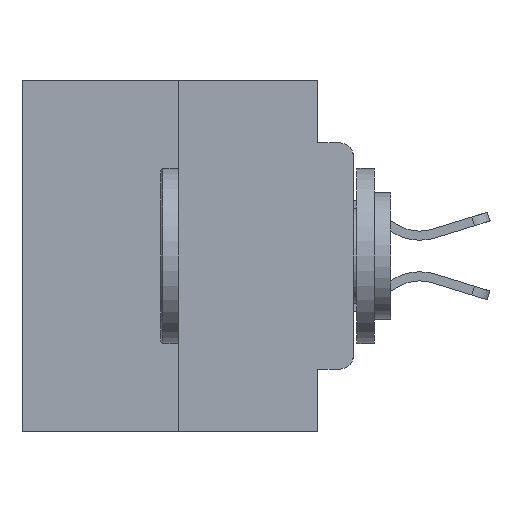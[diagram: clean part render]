
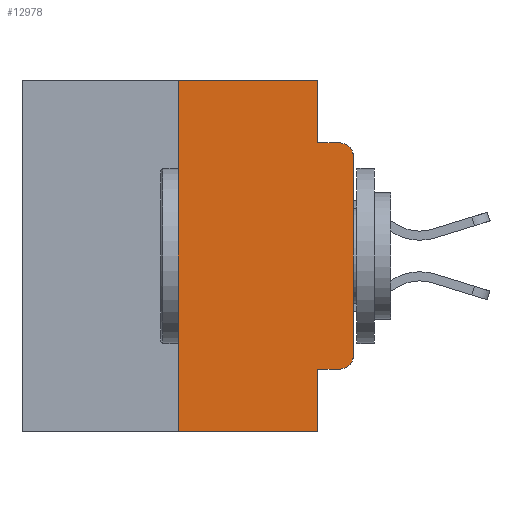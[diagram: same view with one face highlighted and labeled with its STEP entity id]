
A CAD part, left-side view. The second image highlights one B-rep face of the part: STEP entity #12978.
In plain terms, the highlighted planar face has unit normal (-1, 0, 0).
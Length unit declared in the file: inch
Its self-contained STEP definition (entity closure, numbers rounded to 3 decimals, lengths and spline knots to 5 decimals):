
#45 = ORIENTED_EDGE ( 'NONE', *, *, #5260, .T. ) ;
#410 = EDGE_CURVE ( 'NONE', #4877, #18952, #23578, .T. ) ;
#663 = VERTEX_POINT ( 'NONE', #10787 ) ;
#1080 = CARTESIAN_POINT ( 'NONE',  ( 0., 0.02, -0.4115 ) ) ;
#1214 = CIRCLE ( 'NONE', #4079, 0.02 ) ;
#1266 = DIRECTION ( 'NONE',  ( 0., 0., -1. ) ) ;
#1281 = CARTESIAN_POINT ( 'NONE',  ( 0., 0.25, 0. ) ) ;
#1569 = ORIENTED_EDGE ( 'NONE', *, *, #19447, .F. ) ;
#2007 = ORIENTED_EDGE ( 'NONE', *, *, #410, .T. ) ;
#2140 = VERTEX_POINT ( 'NONE', #1281 ) ;
#2347 = VECTOR ( 'NONE', #6789, 39.37008 ) ;
#2609 = ORIENTED_EDGE ( 'NONE', *, *, #10534, .F. ) ;
#2623 = VECTOR ( 'NONE', #26717, 39.37008 ) ;
#2697 = DIRECTION ( 'NONE',  ( 0., -1., 0. ) ) ;
#2991 = CARTESIAN_POINT ( 'NONE',  ( 0., 0.02, -0.1085 ) ) ;
#3119 = ORIENTED_EDGE ( 'NONE', *, *, #18502, .F. ) ;
#3158 = LINE ( 'NONE', #25580, #23714 ) ;
#3335 = CARTESIAN_POINT ( 'NONE',  ( 0., 0.02, -0.0885 ) ) ;
#3342 = VERTEX_POINT ( 'NONE', #7476 ) ;
#3512 = EDGE_LOOP ( 'NONE', ( #21358, #22064, #22658, #17281, #3119, #2609, #2007, #1569, #45, #16520 ) ) ;
#3519 = DIRECTION ( 'NONE',  ( 1., 0., 0. ) ) ;
#3778 = EDGE_CURVE ( 'NONE', #18759, #14320, #3158, .T. ) ;
#4079 = AXIS2_PLACEMENT_3D ( 'NONE', #2991, #17925, #5199 ) ;
#4141 = EDGE_CURVE ( 'NONE', #25461, #663, #26878, .T. ) ;
#4877 = VERTEX_POINT ( 'NONE', #12364 ) ;
#5199 = DIRECTION ( 'NONE',  ( 0., 0., -1. ) ) ;
#5260 = EDGE_CURVE ( 'NONE', #12381, #22173, #23355, .T. ) ;
#5715 = CARTESIAN_POINT ( 'NONE',  ( 0., 0.25, 0. ) ) ;
#5802 = CARTESIAN_POINT ( 'NONE',  ( 0., 0.473, -0.5 ) ) ;
#5827 = CARTESIAN_POINT ( 'NONE',  ( 0., 0.051, 0. ) ) ;
#5860 = CARTESIAN_POINT ( 'NONE',  ( 0., 0.051, -0.0885 ) ) ;
#6789 = DIRECTION ( 'NONE',  ( 0., -1., 0. ) ) ;
#7265 = VECTOR ( 'NONE', #7481, 39.37008 ) ;
#7355 = VECTOR ( 'NONE', #18394, 39.37008 ) ;
#7476 = CARTESIAN_POINT ( 'NONE',  ( 0., 0.051, 0. ) ) ;
#7481 = DIRECTION ( 'NONE',  ( 0., -1., 0. ) ) ;
#8270 = EDGE_CURVE ( 'NONE', #22173, #25461, #11747, .T. ) ;
#8455 = LINE ( 'NONE', #5827, #2623 ) ;
#8773 = CARTESIAN_POINT ( 'NONE',  ( 0., 0.02, -0.3915 ) ) ;
#9856 = VECTOR ( 'NONE', #2697, 39.37008 ) ;
#10022 = CARTESIAN_POINT ( 'NONE',  ( 0., 0.473, 0. ) ) ;
#10534 = EDGE_CURVE ( 'NONE', #4877, #2140, #18562, .T. ) ;
#10787 = CARTESIAN_POINT ( 'NONE',  ( 0., 0., -0.1085 ) ) ;
#10939 = DIRECTION ( 'NONE',  ( 0., 0., -1. ) ) ;
#11041 = EDGE_CURVE ( 'NONE', #663, #14320, #1214, .T. ) ;
#11046 = DIRECTION ( 'NONE',  ( 0., -1., 0. ) ) ;
#11747 = CIRCLE ( 'NONE', #19338, 0.02 ) ;
#12364 = CARTESIAN_POINT ( 'NONE',  ( 0., 0.25, -0.5 ) ) ;
#12381 = VERTEX_POINT ( 'NONE', #14376 ) ;
#12978 = ADVANCED_FACE ( 'NONE', ( #24630 ), #16344, .F. ) ;
#13913 = CARTESIAN_POINT ( 'NONE',  ( 0., 0.051, -0.4115 ) ) ;
#14320 = VERTEX_POINT ( 'NONE', #3335 ) ;
#14376 = CARTESIAN_POINT ( 'NONE',  ( 0., 0.051, -0.4115 ) ) ;
#14987 = CARTESIAN_POINT ( 'NONE',  ( 0., 0.051, -0.5 ) ) ;
#15224 = VECTOR ( 'NONE', #16331, 39.37008 ) ;
#16158 = EDGE_CURVE ( 'NONE', #3342, #18759, #24354, .T. ) ;
#16269 = CARTESIAN_POINT ( 'NONE',  ( 0., 0.051, 0. ) ) ;
#16331 = DIRECTION ( 'NONE',  ( 0., 0., 1. ) ) ;
#16344 = PLANE ( 'NONE',  #20831 ) ;
#16520 = ORIENTED_EDGE ( 'NONE', *, *, #8270, .T. ) ;
#17281 = ORIENTED_EDGE ( 'NONE', *, *, #16158, .F. ) ;
#17925 = DIRECTION ( 'NONE',  ( -1., 0., 0. ) ) ;
#18394 = DIRECTION ( 'NONE',  ( 0., 0., 1. ) ) ;
#18419 = DIRECTION ( 'NONE',  ( 0., 0., -1. ) ) ;
#18502 = EDGE_CURVE ( 'NONE', #2140, #3342, #20982, .T. ) ;
#18562 = LINE ( 'NONE', #5715, #7355 ) ;
#18759 = VERTEX_POINT ( 'NONE', #5860 ) ;
#18822 = VECTOR ( 'NONE', #1266, 39.37008 ) ;
#18952 = VERTEX_POINT ( 'NONE', #14987 ) ;
#19338 = AXIS2_PLACEMENT_3D ( 'NONE', #8773, #23424, #10939 ) ;
#19385 = CARTESIAN_POINT ( 'NONE',  ( 0., 0., -0.3915 ) ) ;
#19447 = EDGE_CURVE ( 'NONE', #12381, #18952, #8455, .T. ) ;
#19638 = CARTESIAN_POINT ( 'NONE',  ( 0., 0.473, 0. ) ) ;
#20831 = AXIS2_PLACEMENT_3D ( 'NONE', #10022, #3519, #18419 ) ;
#20982 = LINE ( 'NONE', #19638, #9856 ) ;
#21358 = ORIENTED_EDGE ( 'NONE', *, *, #4141, .T. ) ;
#22064 = ORIENTED_EDGE ( 'NONE', *, *, #11041, .T. ) ;
#22173 = VERTEX_POINT ( 'NONE', #1080 ) ;
#22658 = ORIENTED_EDGE ( 'NONE', *, *, #3778, .F. ) ;
#23355 = LINE ( 'NONE', #13913, #7265 ) ;
#23424 = DIRECTION ( 'NONE',  ( -1., 0., 0. ) ) ;
#23578 = LINE ( 'NONE', #5802, #2347 ) ;
#23714 = VECTOR ( 'NONE', #11046, 39.37008 ) ;
#24354 = LINE ( 'NONE', #16269, #18822 ) ;
#24630 = FACE_OUTER_BOUND ( 'NONE', #3512, .T. ) ;
#25461 = VERTEX_POINT ( 'NONE', #19385 ) ;
#25580 = CARTESIAN_POINT ( 'NONE',  ( 0., 0.051, -0.0885 ) ) ;
#26709 = CARTESIAN_POINT ( 'NONE',  ( 0., 0., 0. ) ) ;
#26717 = DIRECTION ( 'NONE',  ( 0., 0., -1. ) ) ;
#26878 = LINE ( 'NONE', #26709, #15224 ) ;
